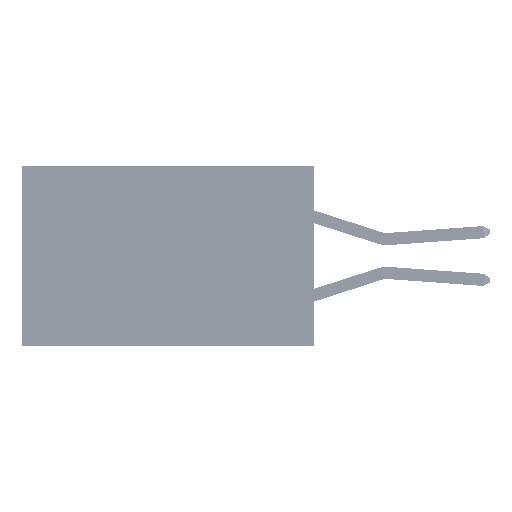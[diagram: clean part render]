
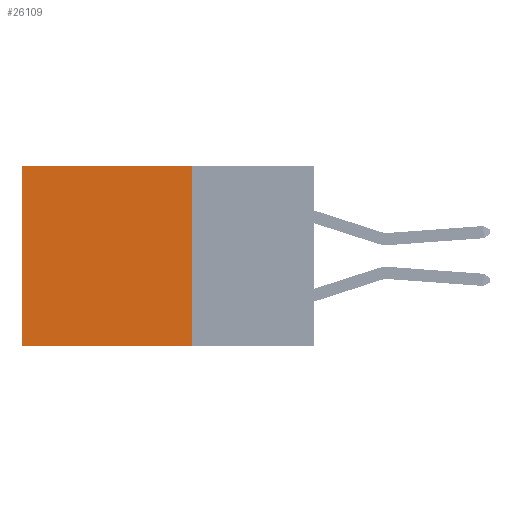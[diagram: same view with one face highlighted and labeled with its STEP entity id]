
A CAD part, left-side view. The second image highlights one B-rep face of the part: STEP entity #26109.
In plain terms, the highlighted planar face has unit normal (-1, 0, 0).
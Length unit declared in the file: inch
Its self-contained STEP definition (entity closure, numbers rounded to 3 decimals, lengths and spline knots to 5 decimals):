
#21 = EDGE_CURVE ( 'NONE', #28759, #9806, #45034, .T. ) ;
#1863 = VECTOR ( 'NONE', #36626, 39.37008 ) ;
#4159 = DIRECTION ( 'NONE',  ( 0., 1., 0. ) ) ;
#7296 = VECTOR ( 'NONE', #4159, 39.37008 ) ;
#8915 = EDGE_LOOP ( 'NONE', ( #34872, #13920, #27846, #27746 ) ) ;
#9806 = VERTEX_POINT ( 'NONE', #30931 ) ;
#10325 = CARTESIAN_POINT ( 'NONE',  ( 0.2875, 0.25, 0. ) ) ;
#11402 = EDGE_CURVE ( 'NONE', #40354, #9806, #38467, .T. ) ;
#11938 = LINE ( 'NONE', #36312, #1863 ) ;
#13441 = DIRECTION ( 'NONE',  ( 0., 0., -1. ) ) ;
#13801 = CARTESIAN_POINT ( 'NONE',  ( 0.2875, 0.25, -0.37 ) ) ;
#13920 = ORIENTED_EDGE ( 'NONE', *, *, #11402, .F. ) ;
#16138 = EDGE_CURVE ( 'NONE', #25343, #28759, #18432, .T. ) ;
#18206 = EDGE_CURVE ( 'NONE', #25343, #40354, #11938, .T. ) ;
#18432 = LINE ( 'NONE', #22051, #47858 ) ;
#18891 = CARTESIAN_POINT ( 'NONE',  ( 0.2875, 0.25, -0.37 ) ) ;
#18912 = CARTESIAN_POINT ( 'NONE',  ( 0.2875, 0.6, 0. ) ) ;
#21511 = PLANE ( 'NONE',  #28714 ) ;
#22051 = CARTESIAN_POINT ( 'NONE',  ( 0.2875, 0.25, 0. ) ) ;
#25036 = CARTESIAN_POINT ( 'NONE',  ( 0.2875, 0.25, 0. ) ) ;
#25343 = VERTEX_POINT ( 'NONE', #25036 ) ;
#26109 = ADVANCED_FACE ( 'NONE', ( #35723 ), #21511, .F. ) ;
#27746 = ORIENTED_EDGE ( 'NONE', *, *, #16138, .T. ) ;
#27846 = ORIENTED_EDGE ( 'NONE', *, *, #18206, .F. ) ;
#28714 = AXIS2_PLACEMENT_3D ( 'NONE', #10325, #36635, #13441 ) ;
#28759 = VERTEX_POINT ( 'NONE', #18912 ) ;
#30931 = CARTESIAN_POINT ( 'NONE',  ( 0.2875, 0.6, -0.37 ) ) ;
#33245 = DIRECTION ( 'NONE',  ( 0., 1., 0. ) ) ;
#34194 = CARTESIAN_POINT ( 'NONE',  ( 0.2875, 0.6, 0. ) ) ;
#34373 = DIRECTION ( 'NONE',  ( 0., 0., -1. ) ) ;
#34872 = ORIENTED_EDGE ( 'NONE', *, *, #21, .T. ) ;
#35723 = FACE_OUTER_BOUND ( 'NONE', #8915, .T. ) ;
#36312 = CARTESIAN_POINT ( 'NONE',  ( 0.2875, 0.25, 0. ) ) ;
#36626 = DIRECTION ( 'NONE',  ( 0., 0., -1. ) ) ;
#36635 = DIRECTION ( 'NONE',  ( 1., 0., 0. ) ) ;
#38467 = LINE ( 'NONE', #18891, #7296 ) ;
#40354 = VERTEX_POINT ( 'NONE', #13801 ) ;
#41509 = VECTOR ( 'NONE', #34373, 39.37008 ) ;
#45034 = LINE ( 'NONE', #34194, #41509 ) ;
#47858 = VECTOR ( 'NONE', #33245, 39.37008 ) ;
